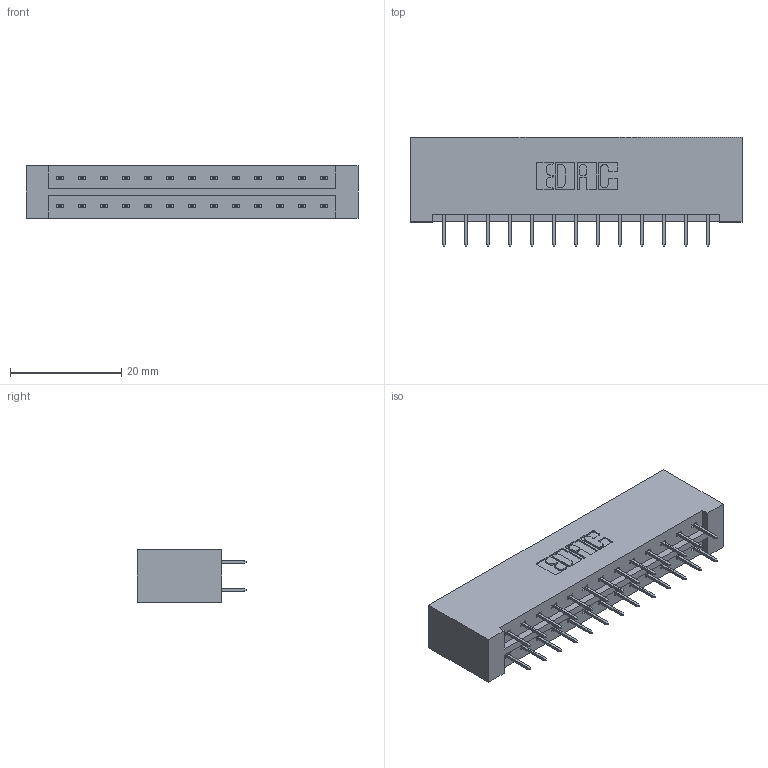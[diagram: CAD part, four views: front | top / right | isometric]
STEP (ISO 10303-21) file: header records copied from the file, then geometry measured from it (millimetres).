
FILE_DESCRIPTION (( 'STEP AP203' ), '1' );
FILE_NAME ('833-026-524-201.STEP', '2020-06-02T04:10:40', ( '' ), ( '' ), 'SwSTEP 2.0', 'SolidWorks 2020', '' );
FILE_SCHEMA (( 'CONFIG_CONTROL_DESIGN' ));
Length unit declared in the file: inch
Products named in the file (3): 833 Part_Lugless; 345-292-001_345-293-124; 833-026-524-201
Assembly tree (27 placements, depth 2):
  833-026-524-201
    833 Part_Lugless
    345-292-001_345-293-124  x26
Bounding box: 59.77 x 19.69 x 9.4 mm (x, y, z)
Volume: 6423.5 mm3; surface area: 7188.8 mm2
Topology: 27 solids, 27 shells, 1562 faces, 4421 edges, 2842 vertices
Faces by surface type: plane 1158, cylinder 404
Entity records: 11911 total; most frequent: CARTESIAN_POINT 2006, ORIENTED_EDGE 1942, DIRECTION 1759, EDGE_CURVE 971, VECTOR 855, LINE 855, VERTEX_POINT 642, AXIS2_PLACEMENT_3D 452
